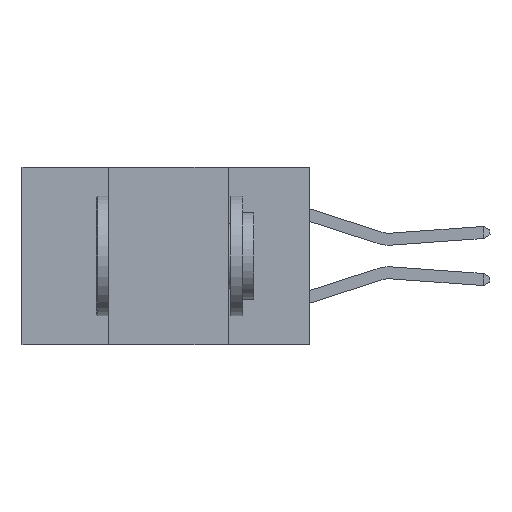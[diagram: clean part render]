
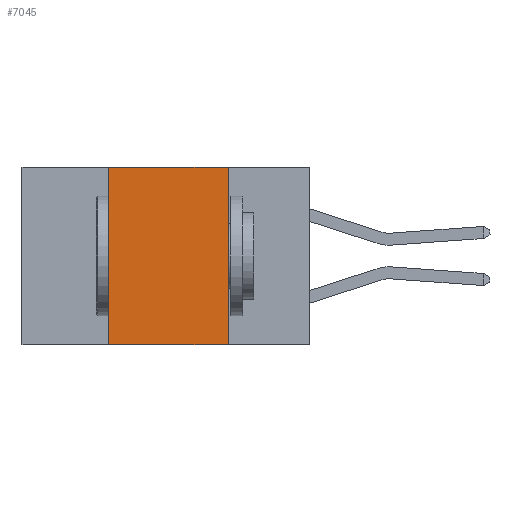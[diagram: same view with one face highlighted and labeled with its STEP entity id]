
A CAD part, left-side view. The second image highlights one B-rep face of the part: STEP entity #7045.
In plain terms, the highlighted planar face has unit normal (-1, 0, 0).
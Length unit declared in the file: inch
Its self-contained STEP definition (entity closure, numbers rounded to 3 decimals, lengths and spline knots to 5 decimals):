
#372 = ORIENTED_EDGE ( 'NONE', *, *, #8096, .F. ) ;
#578 = VERTEX_POINT ( 'NONE', #6119 ) ;
#2668 = CARTESIAN_POINT ( 'NONE',  ( 0., 0.6, -0.37 ) ) ;
#2792 = LINE ( 'NONE', #5196, #5523 ) ;
#2794 = LINE ( 'NONE', #6895, #8029 ) ;
#3352 = ORIENTED_EDGE ( 'NONE', *, *, #4551, .F. ) ;
#3692 = DIRECTION ( 'NONE',  ( 0., 0., 1. ) ) ;
#3808 = VERTEX_POINT ( 'NONE', #10949 ) ;
#4415 = EDGE_LOOP ( 'NONE', ( #372, #5793, #3352, #6143 ) ) ;
#4551 = EDGE_CURVE ( 'NONE', #12337, #578, #13125, .T. ) ;
#5164 = EDGE_CURVE ( 'NONE', #578, #9254, #2792, .T. ) ;
#5196 = CARTESIAN_POINT ( 'NONE',  ( 0., 0.6, 0. ) ) ;
#5523 = VECTOR ( 'NONE', #5885, 39.37008 ) ;
#5793 = ORIENTED_EDGE ( 'NONE', *, *, #5164, .F. ) ;
#5885 = DIRECTION ( 'NONE',  ( 0., -1., 0. ) ) ;
#6119 = CARTESIAN_POINT ( 'NONE',  ( 0., 0.42, 0. ) ) ;
#6143 = ORIENTED_EDGE ( 'NONE', *, *, #11207, .T. ) ;
#6500 = LINE ( 'NONE', #2668, #6825 ) ;
#6825 = VECTOR ( 'NONE', #10045, 39.37008 ) ;
#6834 = FACE_OUTER_BOUND ( 'NONE', #4415, .T. ) ;
#6895 = CARTESIAN_POINT ( 'NONE',  ( 0., 0.17, 0. ) ) ;
#6985 = DIRECTION ( 'NONE',  ( 0., 0., -1. ) ) ;
#7045 = ADVANCED_FACE ( 'NONE', ( #6834 ), #8221, .F. ) ;
#7242 = AXIS2_PLACEMENT_3D ( 'NONE', #7896, #7777, #7737 ) ;
#7737 = DIRECTION ( 'NONE',  ( 0., 0., -1. ) ) ;
#7777 = DIRECTION ( 'NONE',  ( 1., 0., 0. ) ) ;
#7896 = CARTESIAN_POINT ( 'NONE',  ( 0., 0.6, 0. ) ) ;
#8029 = VECTOR ( 'NONE', #6985, 39.37008 ) ;
#8096 = EDGE_CURVE ( 'NONE', #9254, #3808, #2794, .T. ) ;
#8221 = PLANE ( 'NONE',  #7242 ) ;
#8515 = CARTESIAN_POINT ( 'NONE',  ( 0., 0.42, -0.37 ) ) ;
#8599 = CARTESIAN_POINT ( 'NONE',  ( 0., 0.17, 0. ) ) ;
#9254 = VERTEX_POINT ( 'NONE', #8599 ) ;
#10045 = DIRECTION ( 'NONE',  ( 0., -1., 0. ) ) ;
#10070 = VECTOR ( 'NONE', #3692, 39.37008 ) ;
#10949 = CARTESIAN_POINT ( 'NONE',  ( 0., 0.17, -0.37 ) ) ;
#11207 = EDGE_CURVE ( 'NONE', #12337, #3808, #6500, .T. ) ;
#12337 = VERTEX_POINT ( 'NONE', #8515 ) ;
#12566 = CARTESIAN_POINT ( 'NONE',  ( 0., 0.42, 0. ) ) ;
#13125 = LINE ( 'NONE', #12566, #10070 ) ;
